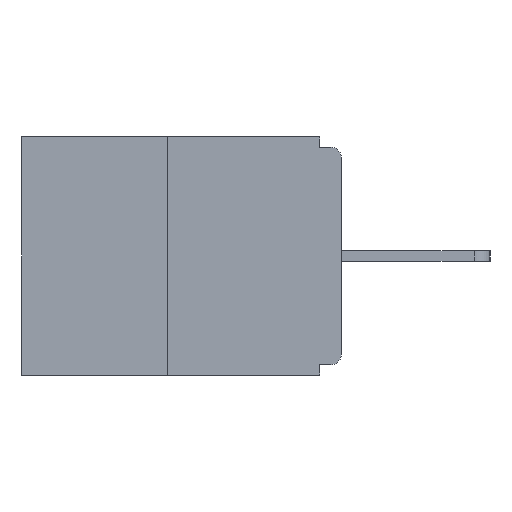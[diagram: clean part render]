
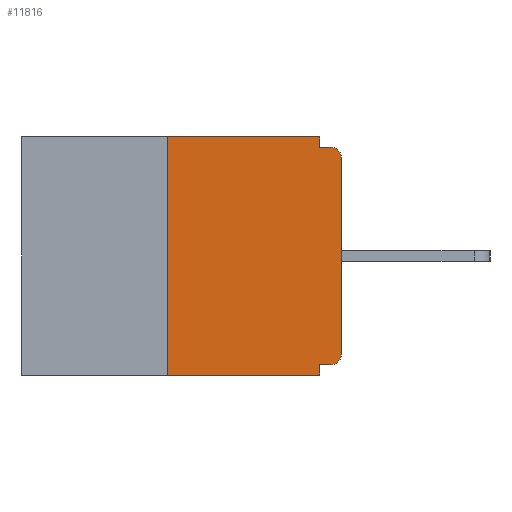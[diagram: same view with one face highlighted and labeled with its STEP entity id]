
A CAD part, left-side view. The second image highlights one B-rep face of the part: STEP entity #11816.
In plain terms, the highlighted planar face has unit normal (-1, 0, 0).
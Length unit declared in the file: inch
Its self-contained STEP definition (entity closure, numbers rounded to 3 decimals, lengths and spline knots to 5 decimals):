
#22 = CARTESIAN_POINT ( 'NONE',  ( 0., 0.46, -0.343 ) ) ;
#140 = EDGE_LOOP ( 'NONE', ( #17713, #3678, #18273, #4269, #14531, #384, #20578, #1600, #7174, #12013 ) ) ;
#375 = AXIS2_PLACEMENT_3D ( 'NONE', #10006, #22760, #11824 ) ;
#384 = ORIENTED_EDGE ( 'NONE', *, *, #23095, .T. ) ;
#436 = DIRECTION ( 'NONE',  ( 0., 0., 1. ) ) ;
#768 = LINE ( 'NONE', #13836, #19807 ) ;
#1061 = VERTEX_POINT ( 'NONE', #12584 ) ;
#1600 = ORIENTED_EDGE ( 'NONE', *, *, #20646, .T. ) ;
#1687 = EDGE_CURVE ( 'NONE', #22335, #2005, #7700, .T. ) ;
#2005 = VERTEX_POINT ( 'NONE', #16736 ) ;
#2530 = LINE ( 'NONE', #13373, #21491 ) ;
#2731 = VECTOR ( 'NONE', #20934, 39.37008 ) ;
#3112 = CARTESIAN_POINT ( 'NONE',  ( 0., 0., -0.015 ) ) ;
#3612 = VERTEX_POINT ( 'NONE', #8216 ) ;
#3678 = ORIENTED_EDGE ( 'NONE', *, *, #12510, .F. ) ;
#4167 = VERTEX_POINT ( 'NONE', #9912 ) ;
#4269 = ORIENTED_EDGE ( 'NONE', *, *, #10097, .F. ) ;
#4385 = VERTEX_POINT ( 'NONE', #12514 ) ;
#4918 = CARTESIAN_POINT ( 'NONE',  ( 0., 0.25, 0. ) ) ;
#5362 = DIRECTION ( 'NONE',  ( 1., 0., 0. ) ) ;
#5707 = DIRECTION ( 'NONE',  ( 0., -1., 0. ) ) ;
#5895 = CIRCLE ( 'NONE', #375, 0.015 ) ;
#6448 = LINE ( 'NONE', #14896, #15506 ) ;
#6701 = CARTESIAN_POINT ( 'NONE',  ( 0., 0.015, -0.03 ) ) ;
#6741 = EDGE_CURVE ( 'NONE', #12982, #14589, #22754, .T. ) ;
#7174 = ORIENTED_EDGE ( 'NONE', *, *, #1687, .F. ) ;
#7203 = EDGE_CURVE ( 'NONE', #8052, #4167, #6448, .T. ) ;
#7403 = DIRECTION ( 'NONE',  ( 0., 0., -1. ) ) ;
#7700 = LINE ( 'NONE', #3112, #2731 ) ;
#7969 = DIRECTION ( 'NONE',  ( 0., 1., 0. ) ) ;
#8052 = VERTEX_POINT ( 'NONE', #4918 ) ;
#8211 = VECTOR ( 'NONE', #7969, 39.37008 ) ;
#8216 = CARTESIAN_POINT ( 'NONE',  ( 0., 0., -0.03 ) ) ;
#8311 = CARTESIAN_POINT ( 'NONE',  ( 0., 0., -0.328 ) ) ;
#8434 = LINE ( 'NONE', #22, #12668 ) ;
#8550 = DIRECTION ( 'NONE',  ( 0., 0., -1. ) ) ;
#8894 = EDGE_CURVE ( 'NONE', #4167, #22335, #19777, .T. ) ;
#8946 = PLANE ( 'NONE',  #17039 ) ;
#9912 = CARTESIAN_POINT ( 'NONE',  ( 0., 0.031, 0. ) ) ;
#9917 = VECTOR ( 'NONE', #13173, 39.37008 ) ;
#10006 = CARTESIAN_POINT ( 'NONE',  ( 0., 0.015, -0.313 ) ) ;
#10097 = EDGE_CURVE ( 'NONE', #14589, #13488, #14692, .T. ) ;
#11311 = EDGE_CURVE ( 'NONE', #4385, #13488, #8434, .T. ) ;
#11525 = FACE_OUTER_BOUND ( 'NONE', #140, .T. ) ;
#11627 = EDGE_CURVE ( 'NONE', #1061, #3612, #768, .T. ) ;
#11816 = ADVANCED_FACE ( 'NONE', ( #11525 ), #8946, .F. ) ;
#11824 = DIRECTION ( 'NONE',  ( 0., 0., -1. ) ) ;
#12013 = ORIENTED_EDGE ( 'NONE', *, *, #8894, .F. ) ;
#12510 = EDGE_CURVE ( 'NONE', #4385, #8052, #2530, .T. ) ;
#12514 = CARTESIAN_POINT ( 'NONE',  ( 0., 0.25, -0.343 ) ) ;
#12584 = CARTESIAN_POINT ( 'NONE',  ( 0., 0., -0.313 ) ) ;
#12668 = VECTOR ( 'NONE', #5707, 39.37008 ) ;
#12982 = VERTEX_POINT ( 'NONE', #14688 ) ;
#13173 = DIRECTION ( 'NONE',  ( 0., 0., -1. ) ) ;
#13373 = CARTESIAN_POINT ( 'NONE',  ( 0., 0.25, 0. ) ) ;
#13488 = VERTEX_POINT ( 'NONE', #19825 ) ;
#13640 = AXIS2_PLACEMENT_3D ( 'NONE', #6701, #19452, #8550 ) ;
#13836 = CARTESIAN_POINT ( 'NONE',  ( 0., 0., 0. ) ) ;
#14531 = ORIENTED_EDGE ( 'NONE', *, *, #6741, .F. ) ;
#14589 = VERTEX_POINT ( 'NONE', #22666 ) ;
#14688 = CARTESIAN_POINT ( 'NONE',  ( 0., 0.015, -0.328 ) ) ;
#14692 = LINE ( 'NONE', #16766, #9917 ) ;
#14857 = VECTOR ( 'NONE', #7403, 39.37008 ) ;
#14896 = CARTESIAN_POINT ( 'NONE',  ( 0., 0.46, 0. ) ) ;
#15506 = VECTOR ( 'NONE', #16764, 39.37008 ) ;
#16267 = CARTESIAN_POINT ( 'NONE',  ( 0., 0.46, 0. ) ) ;
#16736 = CARTESIAN_POINT ( 'NONE',  ( 0., 0.015, -0.015 ) ) ;
#16764 = DIRECTION ( 'NONE',  ( 0., -1., 0. ) ) ;
#16766 = CARTESIAN_POINT ( 'NONE',  ( 0., 0.031, -0.343 ) ) ;
#17039 = AXIS2_PLACEMENT_3D ( 'NONE', #16267, #5362, #18152 ) ;
#17713 = ORIENTED_EDGE ( 'NONE', *, *, #7203, .F. ) ;
#18152 = DIRECTION ( 'NONE',  ( 0., 0., -1. ) ) ;
#18273 = ORIENTED_EDGE ( 'NONE', *, *, #11311, .T. ) ;
#19452 = DIRECTION ( 'NONE',  ( -1., 0., 0. ) ) ;
#19777 = LINE ( 'NONE', #23822, #14857 ) ;
#19807 = VECTOR ( 'NONE', #23052, 39.37008 ) ;
#19825 = CARTESIAN_POINT ( 'NONE',  ( 0., 0.031, -0.343 ) ) ;
#20578 = ORIENTED_EDGE ( 'NONE', *, *, #11627, .T. ) ;
#20625 = CARTESIAN_POINT ( 'NONE',  ( 0., 0.031, -0.015 ) ) ;
#20646 = EDGE_CURVE ( 'NONE', #3612, #2005, #21331, .T. ) ;
#20934 = DIRECTION ( 'NONE',  ( 0., -1., 0. ) ) ;
#21331 = CIRCLE ( 'NONE', #13640, 0.015 ) ;
#21491 = VECTOR ( 'NONE', #436, 39.37008 ) ;
#22335 = VERTEX_POINT ( 'NONE', #20625 ) ;
#22666 = CARTESIAN_POINT ( 'NONE',  ( 0., 0.031, -0.328 ) ) ;
#22754 = LINE ( 'NONE', #8311, #8211 ) ;
#22760 = DIRECTION ( 'NONE',  ( -1., 0., 0. ) ) ;
#23052 = DIRECTION ( 'NONE',  ( 0., 0., 1. ) ) ;
#23095 = EDGE_CURVE ( 'NONE', #12982, #1061, #5895, .T. ) ;
#23822 = CARTESIAN_POINT ( 'NONE',  ( 0., 0.031, 0. ) ) ;
